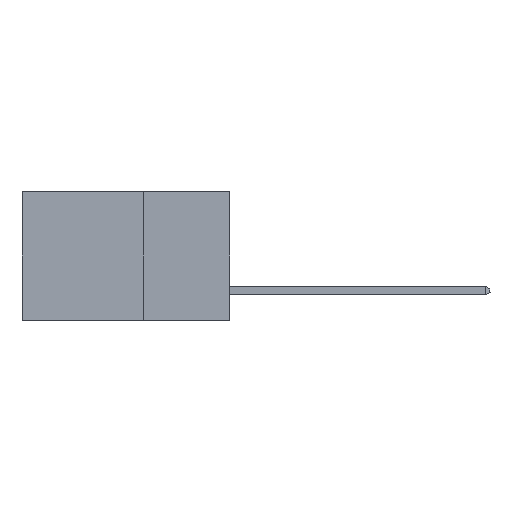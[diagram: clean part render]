
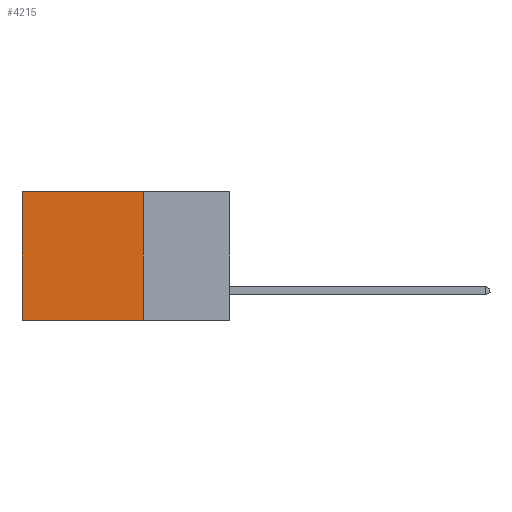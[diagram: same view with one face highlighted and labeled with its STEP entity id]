
A CAD part, left-side view. The second image highlights one B-rep face of the part: STEP entity #4215.
In plain terms, the highlighted planar face has unit normal (-1, 0, 0).
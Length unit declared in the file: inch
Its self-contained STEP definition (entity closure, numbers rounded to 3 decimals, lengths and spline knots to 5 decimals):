
#212 = CARTESIAN_POINT ( 'NONE',  ( 0.298, 0.25, 0. ) ) ;
#2770 = DIRECTION ( 'NONE',  ( 0., 1., 0. ) ) ;
#3586 = EDGE_LOOP ( 'NONE', ( #6467, #9462, #14901, #23307 ) ) ;
#3680 = VERTEX_POINT ( 'NONE', #4673 ) ;
#4215 = ADVANCED_FACE ( 'NONE', ( #15520 ), #10843, .F. ) ;
#4673 = CARTESIAN_POINT ( 'NONE',  ( 0.298, 0.25, -0.37 ) ) ;
#5729 = AXIS2_PLACEMENT_3D ( 'NONE', #212, #8957, #19899 ) ;
#6467 = ORIENTED_EDGE ( 'NONE', *, *, #21272, .T. ) ;
#6636 = VERTEX_POINT ( 'NONE', #21583 ) ;
#6790 = EDGE_CURVE ( 'NONE', #3680, #18711, #18199, .T. ) ;
#7507 = LINE ( 'NONE', #8086, #7773 ) ;
#7773 = VECTOR ( 'NONE', #12026, 39.37008 ) ;
#8047 = VERTEX_POINT ( 'NONE', #19851 ) ;
#8086 = CARTESIAN_POINT ( 'NONE',  ( 0.298, 0.25, 0. ) ) ;
#8957 = DIRECTION ( 'NONE',  ( 1., 0., 0. ) ) ;
#9045 = VECTOR ( 'NONE', #21536, 39.37008 ) ;
#9167 = DIRECTION ( 'NONE',  ( 0., 0., -1. ) ) ;
#9462 = ORIENTED_EDGE ( 'NONE', *, *, #6790, .F. ) ;
#9590 = CARTESIAN_POINT ( 'NONE',  ( 0.298, 0.6, 0. ) ) ;
#9604 = CARTESIAN_POINT ( 'NONE',  ( 0.298, 0.25, -0.37 ) ) ;
#10843 = PLANE ( 'NONE',  #5729 ) ;
#12026 = DIRECTION ( 'NONE',  ( 0., 1., 0. ) ) ;
#14901 = ORIENTED_EDGE ( 'NONE', *, *, #21071, .F. ) ;
#15423 = CARTESIAN_POINT ( 'NONE',  ( 0.298, 0.25, 0. ) ) ;
#15520 = FACE_OUTER_BOUND ( 'NONE', #3586, .T. ) ;
#16719 = VECTOR ( 'NONE', #2770, 39.37008 ) ;
#18199 = LINE ( 'NONE', #9604, #16719 ) ;
#18339 = LINE ( 'NONE', #9590, #23459 ) ;
#18711 = VERTEX_POINT ( 'NONE', #21169 ) ;
#19851 = CARTESIAN_POINT ( 'NONE',  ( 0.298, 0.6, 0. ) ) ;
#19899 = DIRECTION ( 'NONE',  ( 0., 0., -1. ) ) ;
#21071 = EDGE_CURVE ( 'NONE', #6636, #3680, #26048, .T. ) ;
#21169 = CARTESIAN_POINT ( 'NONE',  ( 0.298, 0.6, -0.37 ) ) ;
#21272 = EDGE_CURVE ( 'NONE', #8047, #18711, #18339, .T. ) ;
#21536 = DIRECTION ( 'NONE',  ( 0., 0., -1. ) ) ;
#21583 = CARTESIAN_POINT ( 'NONE',  ( 0.298, 0.25, 0. ) ) ;
#23307 = ORIENTED_EDGE ( 'NONE', *, *, #24270, .T. ) ;
#23459 = VECTOR ( 'NONE', #9167, 39.37008 ) ;
#24270 = EDGE_CURVE ( 'NONE', #6636, #8047, #7507, .T. ) ;
#26048 = LINE ( 'NONE', #15423, #9045 ) ;
